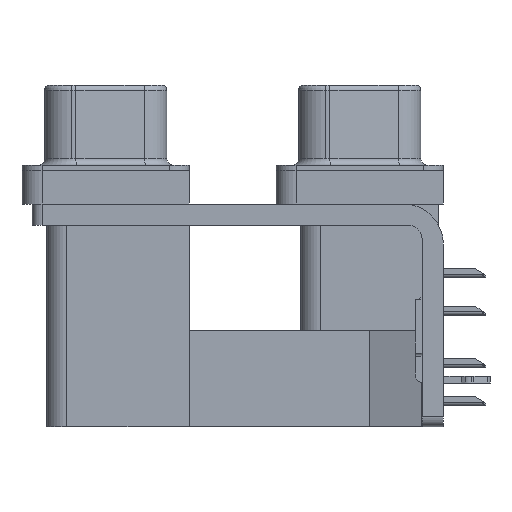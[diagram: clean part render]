
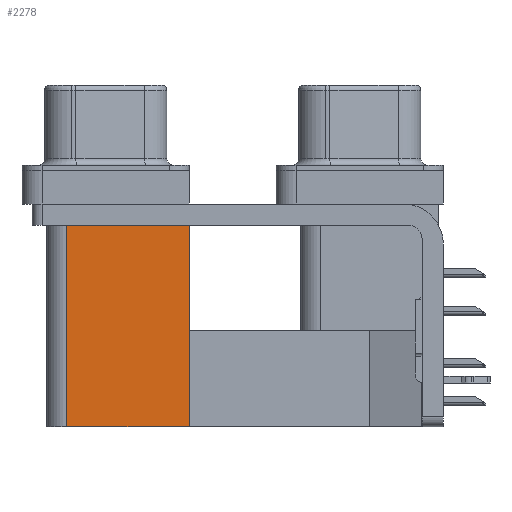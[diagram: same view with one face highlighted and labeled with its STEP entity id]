
A CAD part, left-side view. The second image highlights one B-rep face of the part: STEP entity #2278.
In plain terms, the highlighted planar face has unit normal (-1, 0, 0).
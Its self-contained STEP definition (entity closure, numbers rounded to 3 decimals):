
#724 = LINE ( 'NONE', #20016, #13442 ) ;
#1838 = VECTOR ( 'NONE', #1860, 1000. ) ;
#1851 = EDGE_CURVE ( 'NONE', #25642, #5598, #21163, .T. ) ;
#1860 = DIRECTION ( 'NONE',  ( 0., 0., 1. ) ) ;
#2075 = ORIENTED_EDGE ( 'NONE', *, *, #1851, .T. ) ;
#2157 = ORIENTED_EDGE ( 'NONE', *, *, #9089, .F. ) ;
#2278 = ADVANCED_FACE ( 'NONE', ( #7242 ), #26573, .F. ) ;
#3339 = EDGE_CURVE ( 'NONE', #8717, #5598, #4378, .T. ) ;
#4378 = LINE ( 'NONE', #19475, #10598 ) ;
#5598 = VERTEX_POINT ( 'NONE', #17191 ) ;
#6067 = CARTESIAN_POINT ( 'NONE',  ( 3.79, 21.975, -19.2 ) ) ;
#7242 = FACE_OUTER_BOUND ( 'NONE', #13146, .T. ) ;
#7518 = DIRECTION ( 'NONE',  ( 0., 1., 0. ) ) ;
#8717 = VERTEX_POINT ( 'NONE', #6067 ) ;
#9089 = EDGE_CURVE ( 'NONE', #18481, #8717, #724, .T. ) ;
#10598 = VECTOR ( 'NONE', #11072, 1000. ) ;
#11072 = DIRECTION ( 'NONE',  ( 0., 0., 1. ) ) ;
#12624 = LINE ( 'NONE', #25363, #1838 ) ;
#13146 = EDGE_LOOP ( 'NONE', ( #2075, #20244, #2157, #19035 ) ) ;
#13442 = VECTOR ( 'NONE', #18086, 1000. ) ;
#13533 = CARTESIAN_POINT ( 'NONE',  ( 3.79, 12.775, -19.2 ) ) ;
#16158 = AXIS2_PLACEMENT_3D ( 'NONE', #13533, #17735, #7518 ) ;
#16711 = CARTESIAN_POINT ( 'NONE',  ( 3.79, 12.775, -2.5 ) ) ;
#17191 = CARTESIAN_POINT ( 'NONE',  ( 3.79, 21.975, -2.5 ) ) ;
#17357 = DIRECTION ( 'NONE',  ( 0., 1., 0. ) ) ;
#17502 = CARTESIAN_POINT ( 'NONE',  ( 3.79, 12.775, -2.5 ) ) ;
#17735 = DIRECTION ( 'NONE',  ( 1., 0., 0. ) ) ;
#18086 = DIRECTION ( 'NONE',  ( 0., 1., 0. ) ) ;
#18481 = VERTEX_POINT ( 'NONE', #20818 ) ;
#19035 = ORIENTED_EDGE ( 'NONE', *, *, #22478, .T. ) ;
#19475 = CARTESIAN_POINT ( 'NONE',  ( 3.79, 21.975, -19.2 ) ) ;
#20016 = CARTESIAN_POINT ( 'NONE',  ( 3.79, 12.775, -19.2 ) ) ;
#20244 = ORIENTED_EDGE ( 'NONE', *, *, #3339, .F. ) ;
#20818 = CARTESIAN_POINT ( 'NONE',  ( 3.79, 12.775, -19.2 ) ) ;
#21163 = LINE ( 'NONE', #17502, #23037 ) ;
#22478 = EDGE_CURVE ( 'NONE', #18481, #25642, #12624, .T. ) ;
#23037 = VECTOR ( 'NONE', #17357, 1000. ) ;
#25363 = CARTESIAN_POINT ( 'NONE',  ( 3.79, 12.775, -19.2 ) ) ;
#25642 = VERTEX_POINT ( 'NONE', #16711 ) ;
#26573 = PLANE ( 'NONE',  #16158 ) ;
